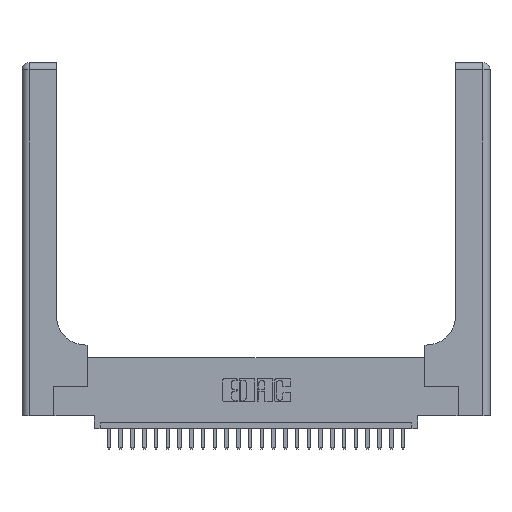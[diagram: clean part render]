
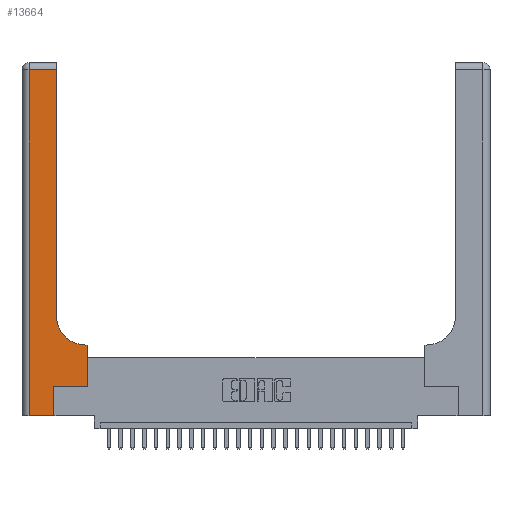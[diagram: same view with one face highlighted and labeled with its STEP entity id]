
A CAD part, top view. The second image highlights one B-rep face of the part: STEP entity #13664.
In plain terms, the highlighted planar face has unit normal (0, 0, 1).
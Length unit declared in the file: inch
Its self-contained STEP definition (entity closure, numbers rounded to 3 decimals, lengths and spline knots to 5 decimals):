
#12 = FACE_OUTER_BOUND ( 'NONE', #18773, .T. ) ;
#946 = DIRECTION ( 'NONE',  ( -1., 0., 0. ) ) ;
#1002 = VERTEX_POINT ( 'NONE', #25007 ) ;
#1122 = DIRECTION ( 'NONE',  ( 1., 0., 0. ) ) ;
#1297 = CARTESIAN_POINT ( 'NONE',  ( 0.269, 0.25, 0.37 ) ) ;
#1350 = CARTESIAN_POINT ( 'NONE',  ( 0.2915, 0.6, 0.37 ) ) ;
#1374 = VERTEX_POINT ( 'NONE', #5203 ) ;
#1509 = DIRECTION ( 'NONE',  ( 1., 0., 0. ) ) ;
#1652 = AXIS2_PLACEMENT_3D ( 'NONE', #15636, #6988, #946 ) ;
#1833 = ORIENTED_EDGE ( 'NONE', *, *, #26300, .T. ) ;
#2898 = CARTESIAN_POINT ( 'NONE',  ( 0.06, 0., 0.37 ) ) ;
#3251 = DIRECTION ( 'NONE',  ( 0., 1., 0. ) ) ;
#3528 = CARTESIAN_POINT ( 'NONE',  ( 0.5585, 0.25, 0.37 ) ) ;
#3723 = CARTESIAN_POINT ( 'NONE',  ( 0.269, 0., 0.37 ) ) ;
#4680 = LINE ( 'NONE', #1350, #11577 ) ;
#5203 = CARTESIAN_POINT ( 'NONE',  ( 0.2915, 0.85, 0.37 ) ) ;
#5293 = ORIENTED_EDGE ( 'NONE', *, *, #26177, .T. ) ;
#5371 = CARTESIAN_POINT ( 'NONE',  ( 0.2915, 2.94, 0.37 ) ) ;
#5389 = EDGE_CURVE ( 'NONE', #22446, #16116, #18875, .T. ) ;
#5623 = ORIENTED_EDGE ( 'NONE', *, *, #16079, .T. ) ;
#6322 = VERTEX_POINT ( 'NONE', #21149 ) ;
#6904 = ORIENTED_EDGE ( 'NONE', *, *, #14061, .T. ) ;
#6988 = DIRECTION ( 'NONE',  ( 0., 0., -1. ) ) ;
#7347 = DIRECTION ( 'NONE',  ( 0., 0., -1. ) ) ;
#7674 = ORIENTED_EDGE ( 'NONE', *, *, #20263, .T. ) ;
#8860 = ORIENTED_EDGE ( 'NONE', *, *, #5389, .T. ) ;
#8960 = ORIENTED_EDGE ( 'NONE', *, *, #24961, .T. ) ;
#9641 = VECTOR ( 'NONE', #19050, 39.37008 ) ;
#10444 = CARTESIAN_POINT ( 'NONE',  ( 0.06, 3., 0.37 ) ) ;
#10659 = LINE ( 'NONE', #23170, #9641 ) ;
#11577 = VECTOR ( 'NONE', #16143, 39.37008 ) ;
#11777 = VECTOR ( 'NONE', #22880, 39.37008 ) ;
#12029 = CARTESIAN_POINT ( 'NONE',  ( 0., 0., 0.37 ) ) ;
#12031 = CARTESIAN_POINT ( 'NONE',  ( 0.5415, 0.6, 0.37 ) ) ;
#12369 = LINE ( 'NONE', #12029, #27151 ) ;
#12941 = ORIENTED_EDGE ( 'NONE', *, *, #23030, .T. ) ;
#13272 = VECTOR ( 'NONE', #16163, 39.37008 ) ;
#13664 = ADVANCED_FACE ( 'NONE', ( #12 ), #15267, .F. ) ;
#14061 = EDGE_CURVE ( 'NONE', #1002, #16006, #17301, .T. ) ;
#15027 = EDGE_CURVE ( 'NONE', #16006, #6322, #12369, .T. ) ;
#15267 = PLANE ( 'NONE',  #1652 ) ;
#15636 = CARTESIAN_POINT ( 'NONE',  ( 0., 3., 0.37 ) ) ;
#16006 = VERTEX_POINT ( 'NONE', #2898 ) ;
#16079 = EDGE_CURVE ( 'NONE', #16116, #16737, #17878, .T. ) ;
#16116 = VERTEX_POINT ( 'NONE', #3528 ) ;
#16122 = CARTESIAN_POINT ( 'NONE',  ( 0.2915, 3., 0.37 ) ) ;
#16143 = DIRECTION ( 'NONE',  ( -1., 0., 0. ) ) ;
#16163 = DIRECTION ( 'NONE',  ( 1., 0., 0. ) ) ;
#16737 = VERTEX_POINT ( 'NONE', #25384 ) ;
#17301 = LINE ( 'NONE', #10444, #11777 ) ;
#17878 = LINE ( 'NONE', #20284, #21488 ) ;
#17885 = LINE ( 'NONE', #3723, #22161 ) ;
#17892 = DIRECTION ( 'NONE',  ( 0., 1., 0. ) ) ;
#18773 = EDGE_LOOP ( 'NONE', ( #7674, #5293, #6904, #21607, #8960, #8860, #5623, #12941, #1833 ) ) ;
#18875 = LINE ( 'NONE', #24419, #13272 ) ;
#19006 = VERTEX_POINT ( 'NONE', #5371 ) ;
#19050 = DIRECTION ( 'NONE',  ( -1., 0., 0. ) ) ;
#19171 = CIRCLE ( 'NONE', #21005, 0.25 ) ;
#20263 = EDGE_CURVE ( 'NONE', #1374, #19006, #27145, .T. ) ;
#20284 = CARTESIAN_POINT ( 'NONE',  ( 0.5585, 0.25, 0.37 ) ) ;
#21005 = AXIS2_PLACEMENT_3D ( 'NONE', #23891, #7347, #1122 ) ;
#21149 = CARTESIAN_POINT ( 'NONE',  ( 0.269, 0., 0.37 ) ) ;
#21488 = VECTOR ( 'NONE', #17892, 39.37008 ) ;
#21607 = ORIENTED_EDGE ( 'NONE', *, *, #15027, .T. ) ;
#22161 = VECTOR ( 'NONE', #22668, 39.37008 ) ;
#22446 = VERTEX_POINT ( 'NONE', #1297 ) ;
#22668 = DIRECTION ( 'NONE',  ( 0., 1., 0. ) ) ;
#22880 = DIRECTION ( 'NONE',  ( 0., -1., 0. ) ) ;
#23030 = EDGE_CURVE ( 'NONE', #16737, #26058, #4680, .T. ) ;
#23170 = CARTESIAN_POINT ( 'NONE',  ( 0., 2.94, 0.37 ) ) ;
#23891 = CARTESIAN_POINT ( 'NONE',  ( 0.5415, 0.85, 0.37 ) ) ;
#24419 = CARTESIAN_POINT ( 'NONE',  ( 0.269, 0.25, 0.37 ) ) ;
#24961 = EDGE_CURVE ( 'NONE', #6322, #22446, #17885, .T. ) ;
#25007 = CARTESIAN_POINT ( 'NONE',  ( 0.06, 2.94, 0.37 ) ) ;
#25384 = CARTESIAN_POINT ( 'NONE',  ( 0.5585, 0.6, 0.37 ) ) ;
#25475 = VECTOR ( 'NONE', #3251, 39.37008 ) ;
#26058 = VERTEX_POINT ( 'NONE', #12031 ) ;
#26177 = EDGE_CURVE ( 'NONE', #19006, #1002, #10659, .T. ) ;
#26300 = EDGE_CURVE ( 'NONE', #26058, #1374, #19171, .T. ) ;
#27145 = LINE ( 'NONE', #16122, #25475 ) ;
#27151 = VECTOR ( 'NONE', #1509, 39.37008 ) ;
